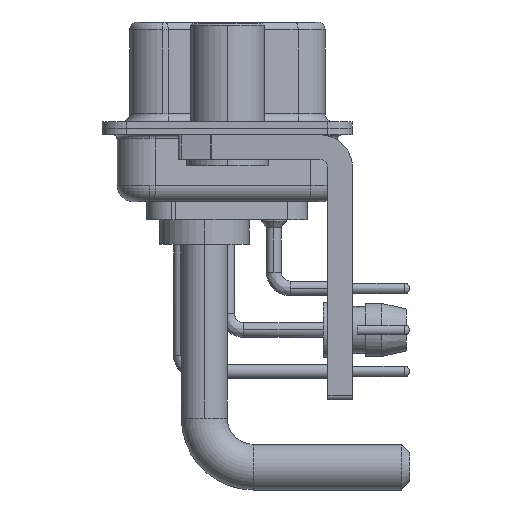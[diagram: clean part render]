
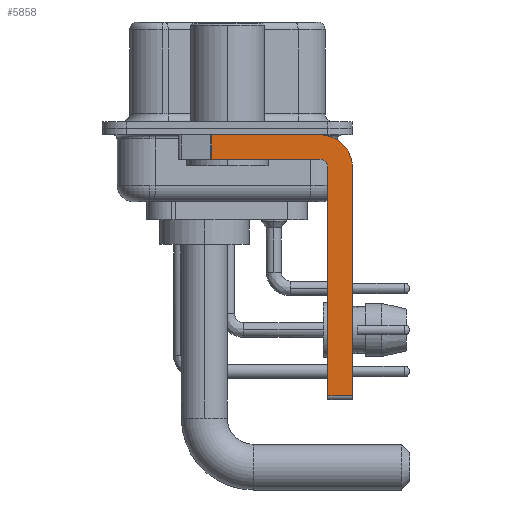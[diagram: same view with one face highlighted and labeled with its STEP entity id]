
A CAD part, left-side view. The second image highlights one B-rep face of the part: STEP entity #5858.
In plain terms, the highlighted planar face has unit normal (-1, 0, 0).
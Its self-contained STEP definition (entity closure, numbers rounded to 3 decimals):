
#1744 = EDGE_CURVE ( 'NONE', #5368, #21358, #27249, .T. ) ;
#2302 = VECTOR ( 'NONE', #21121, 1000. ) ;
#2343 = ORIENTED_EDGE ( 'NONE', *, *, #6830, .F. ) ;
#2576 = ORIENTED_EDGE ( 'NONE', *, *, #3844, .F. ) ;
#3148 = EDGE_CURVE ( 'NONE', #13665, #15354, #9196, .T. ) ;
#3329 = FACE_OUTER_BOUND ( 'NONE', #23003, .T. ) ;
#3753 = CIRCLE ( 'NONE', #34876, 2. ) ;
#3844 = EDGE_CURVE ( 'NONE', #19952, #17312, #3753, .T. ) ;
#4465 = VECTOR ( 'NONE', #31742, 1000. ) ;
#5368 = VERTEX_POINT ( 'NONE', #14459 ) ;
#5417 = ORIENTED_EDGE ( 'NONE', *, *, #1744, .T. ) ;
#5577 = DIRECTION ( 'NONE',  ( 0., 0., -1. ) ) ;
#5723 = CARTESIAN_POINT ( 'NONE',  ( -2.9, -5.65, -16.35 ) ) ;
#5858 = ADVANCED_FACE ( 'NONE', ( #3329 ), #34863, .F. ) ;
#6106 = CARTESIAN_POINT ( 'NONE',  ( -2.9, -7.65, -16.35 ) ) ;
#6830 = EDGE_CURVE ( 'NONE', #15354, #21358, #14703, .T. ) ;
#9077 = DIRECTION ( 'NONE',  ( 0., 0., -1. ) ) ;
#9196 = CIRCLE ( 'NONE', #31761, 0.5 ) ;
#9894 = VERTEX_POINT ( 'NONE', #21288 ) ;
#10113 = VECTOR ( 'NONE', #32606, 1000. ) ;
#10512 = EDGE_CURVE ( 'NONE', #9894, #13665, #10556, .T. ) ;
#10556 = LINE ( 'NONE', #36718, #33189 ) ;
#11988 = CARTESIAN_POINT ( 'NONE',  ( -2.9, 0.978, -1.9 ) ) ;
#12177 = ORIENTED_EDGE ( 'NONE', *, *, #37723, .F. ) ;
#13665 = VERTEX_POINT ( 'NONE', #32743 ) ;
#13878 = CARTESIAN_POINT ( 'NONE',  ( -2.9, -7.65, -2.4 ) ) ;
#13990 = DIRECTION ( 'NONE',  ( 1., 0., 0. ) ) ;
#14419 = ORIENTED_EDGE ( 'NONE', *, *, #24362, .F. ) ;
#14459 = CARTESIAN_POINT ( 'NONE',  ( -2.9, 0.978, -0.4 ) ) ;
#14703 = LINE ( 'NONE', #20418, #29750 ) ;
#14997 = ORIENTED_EDGE ( 'NONE', *, *, #10512, .F. ) ;
#15354 = VERTEX_POINT ( 'NONE', #23451 ) ;
#16269 = DIRECTION ( 'NONE',  ( 0., 0., 1. ) ) ;
#17312 = VERTEX_POINT ( 'NONE', #13878 ) ;
#18435 = ORIENTED_EDGE ( 'NONE', *, *, #27403, .T. ) ;
#18638 = CARTESIAN_POINT ( 'NONE',  ( -2.9, 3., -0.4 ) ) ;
#19952 = VERTEX_POINT ( 'NONE', #28836 ) ;
#20048 = DIRECTION ( 'NONE',  ( 0., 1., 0. ) ) ;
#20081 = LINE ( 'NONE', #34608, #4465 ) ;
#20319 = CARTESIAN_POINT ( 'NONE',  ( -2.9, -5.65, -2.4 ) ) ;
#20418 = CARTESIAN_POINT ( 'NONE',  ( -2.9, -5.65, -1.9 ) ) ;
#20424 = DIRECTION ( 'NONE',  ( 0., -1., 0. ) ) ;
#21121 = DIRECTION ( 'NONE',  ( 0., 0., -1. ) ) ;
#21288 = CARTESIAN_POINT ( 'NONE',  ( -2.9, -6.15, -16.35 ) ) ;
#21358 = VERTEX_POINT ( 'NONE', #22628 ) ;
#22628 = CARTESIAN_POINT ( 'NONE',  ( -2.9, 0.978, -1.9 ) ) ;
#23003 = EDGE_LOOP ( 'NONE', ( #14419, #5417, #2343, #25360, #14997, #18435, #12177, #2576 ) ) ;
#23063 = VECTOR ( 'NONE', #20424, 1000. ) ;
#23451 = CARTESIAN_POINT ( 'NONE',  ( -2.9, -5.65, -1.9 ) ) ;
#24184 = DIRECTION ( 'NONE',  ( -1., 0., 0. ) ) ;
#24362 = EDGE_CURVE ( 'NONE', #5368, #19952, #26880, .T. ) ;
#24373 = CARTESIAN_POINT ( 'NONE',  ( -2.9, -5.65, -2.4 ) ) ;
#25360 = ORIENTED_EDGE ( 'NONE', *, *, #3148, .F. ) ;
#25465 = CARTESIAN_POINT ( 'NONE',  ( -2.9, -5.65, -2.4 ) ) ;
#26689 = DIRECTION ( 'NONE',  ( 0., 0., 1. ) ) ;
#26880 = LINE ( 'NONE', #18638, #10113 ) ;
#27249 = LINE ( 'NONE', #11988, #2302 ) ;
#27403 = EDGE_CURVE ( 'NONE', #9894, #27496, #34045, .T. ) ;
#27496 = VERTEX_POINT ( 'NONE', #6106 ) ;
#28836 = CARTESIAN_POINT ( 'NONE',  ( -2.9, -5.65, -0.4 ) ) ;
#28950 = AXIS2_PLACEMENT_3D ( 'NONE', #20319, #31987, #9077 ) ;
#29750 = VECTOR ( 'NONE', #20048, 1000. ) ;
#31742 = DIRECTION ( 'NONE',  ( 0., 0., -1. ) ) ;
#31761 = AXIS2_PLACEMENT_3D ( 'NONE', #24373, #24184, #26689 ) ;
#31987 = DIRECTION ( 'NONE',  ( 1., 0., 0. ) ) ;
#32606 = DIRECTION ( 'NONE',  ( 0., -1., 0. ) ) ;
#32743 = CARTESIAN_POINT ( 'NONE',  ( -2.9, -6.15, -2.4 ) ) ;
#33189 = VECTOR ( 'NONE', #16269, 1000. ) ;
#34045 = LINE ( 'NONE', #5723, #23063 ) ;
#34608 = CARTESIAN_POINT ( 'NONE',  ( -2.9, -7.65, -2.4 ) ) ;
#34863 = PLANE ( 'NONE',  #28950 ) ;
#34876 = AXIS2_PLACEMENT_3D ( 'NONE', #25465, #13990, #5577 ) ;
#36718 = CARTESIAN_POINT ( 'NONE',  ( -2.9, -6.15, -16.6 ) ) ;
#37723 = EDGE_CURVE ( 'NONE', #17312, #27496, #20081, .T. ) ;
